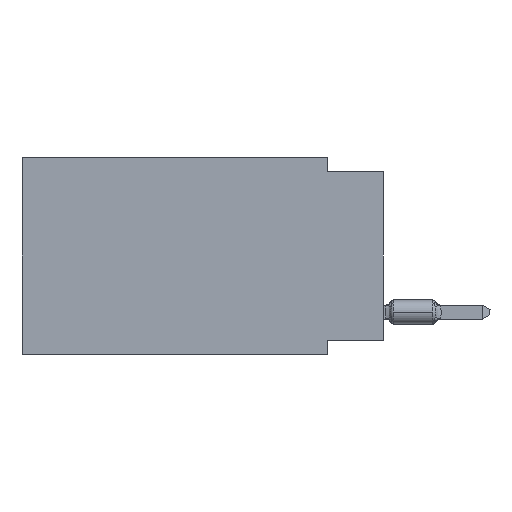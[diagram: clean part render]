
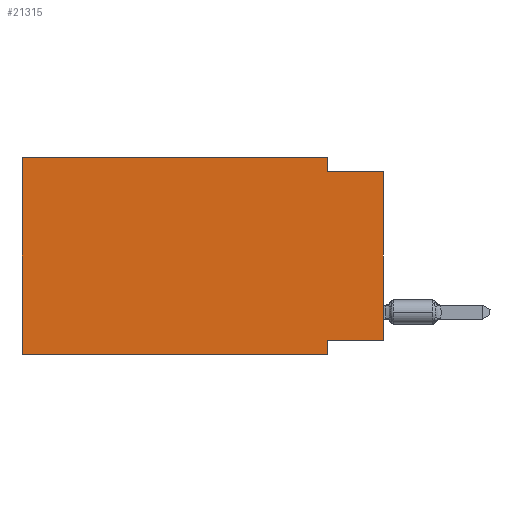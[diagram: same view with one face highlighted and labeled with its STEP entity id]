
A CAD part, left-side view. The second image highlights one B-rep face of the part: STEP entity #21315.
In plain terms, the highlighted planar face has unit normal (-1, 0, 0).
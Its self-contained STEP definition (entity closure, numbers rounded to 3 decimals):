
#63 = LINE ( 'NONE', #19021, #19771 ) ;
#945 = EDGE_CURVE ( 'NONE', #14390, #11680, #5071, .T. ) ;
#1278 = CARTESIAN_POINT ( 'NONE',  ( 0., 2.54, 0. ) ) ;
#1312 = LINE ( 'NONE', #8321, #14700 ) ;
#1321 = VECTOR ( 'NONE', #10752, 1000. ) ;
#1586 = CARTESIAN_POINT ( 'NONE',  ( 0., 0., -8.255 ) ) ;
#1684 = EDGE_CURVE ( 'NONE', #5217, #11494, #1312, .T. ) ;
#1720 = LINE ( 'NONE', #9074, #8133 ) ;
#1744 = DIRECTION ( 'NONE',  ( 0., -1., 0. ) ) ;
#2121 = VERTEX_POINT ( 'NONE', #20463 ) ;
#2567 = CARTESIAN_POINT ( 'NONE',  ( 0., 2.54, -8.89 ) ) ;
#4144 = CARTESIAN_POINT ( 'NONE',  ( 0., 16.383, 0. ) ) ;
#4177 = LINE ( 'NONE', #11512, #22068 ) ;
#4469 = PLANE ( 'NONE',  #6985 ) ;
#4640 = EDGE_CURVE ( 'NONE', #11680, #2121, #7028, .T. ) ;
#4866 = ORIENTED_EDGE ( 'NONE', *, *, #945, .F. ) ;
#5071 = LINE ( 'NONE', #1278, #19088 ) ;
#5217 = VERTEX_POINT ( 'NONE', #13508 ) ;
#6881 = DIRECTION ( 'NONE',  ( 0., -1., 0. ) ) ;
#6985 = AXIS2_PLACEMENT_3D ( 'NONE', #19994, #21599, #14577 ) ;
#7003 = LINE ( 'NONE', #8970, #14429 ) ;
#7018 = EDGE_CURVE ( 'NONE', #5217, #18439, #14177, .T. ) ;
#7028 = LINE ( 'NONE', #10482, #18991 ) ;
#7826 = VERTEX_POINT ( 'NONE', #1586 ) ;
#8072 = EDGE_LOOP ( 'NONE', ( #11065, #15018, #4866, #20286, #22439, #21670, #13181, #9648 ) ) ;
#8133 = VECTOR ( 'NONE', #6881, 1000. ) ;
#8321 = CARTESIAN_POINT ( 'NONE',  ( 0., 16.383, -8.89 ) ) ;
#8581 = DIRECTION ( 'NONE',  ( 0., 1., 0. ) ) ;
#8970 = CARTESIAN_POINT ( 'NONE',  ( 0., 2.54, -8.89 ) ) ;
#9074 = CARTESIAN_POINT ( 'NONE',  ( 0., 16.383, 0. ) ) ;
#9316 = FACE_OUTER_BOUND ( 'NONE', #8072, .T. ) ;
#9648 = ORIENTED_EDGE ( 'NONE', *, *, #9700, .F. ) ;
#9700 = EDGE_CURVE ( 'NONE', #7826, #15382, #63, .T. ) ;
#10275 = DIRECTION ( 'NONE',  ( 0., -1., 0. ) ) ;
#10283 = CARTESIAN_POINT ( 'NONE',  ( 0., 2.54, 0. ) ) ;
#10482 = CARTESIAN_POINT ( 'NONE',  ( 0., 0., -0.635 ) ) ;
#10752 = DIRECTION ( 'NONE',  ( 0., 0., 1. ) ) ;
#11065 = ORIENTED_EDGE ( 'NONE', *, *, #22175, .T. ) ;
#11494 = VERTEX_POINT ( 'NONE', #2567 ) ;
#11512 = CARTESIAN_POINT ( 'NONE',  ( 0., 0., 0. ) ) ;
#11680 = VERTEX_POINT ( 'NONE', #22098 ) ;
#12067 = DIRECTION ( 'NONE',  ( 0., 0., -1. ) ) ;
#13181 = ORIENTED_EDGE ( 'NONE', *, *, #15806, .F. ) ;
#13508 = CARTESIAN_POINT ( 'NONE',  ( 0., 16.383, -8.89 ) ) ;
#13555 = EDGE_CURVE ( 'NONE', #18439, #14390, #1720, .T. ) ;
#14177 = LINE ( 'NONE', #17755, #1321 ) ;
#14390 = VERTEX_POINT ( 'NONE', #10283 ) ;
#14429 = VECTOR ( 'NONE', #21027, 1000. ) ;
#14577 = DIRECTION ( 'NONE',  ( 0., 0., -1. ) ) ;
#14700 = VECTOR ( 'NONE', #10275, 1000. ) ;
#15018 = ORIENTED_EDGE ( 'NONE', *, *, #4640, .F. ) ;
#15382 = VERTEX_POINT ( 'NONE', #21794 ) ;
#15806 = EDGE_CURVE ( 'NONE', #15382, #11494, #7003, .T. ) ;
#17755 = CARTESIAN_POINT ( 'NONE',  ( 0., 16.383, 0. ) ) ;
#18439 = VERTEX_POINT ( 'NONE', #4144 ) ;
#18991 = VECTOR ( 'NONE', #1744, 1000. ) ;
#19021 = CARTESIAN_POINT ( 'NONE',  ( 0., 0., -8.255 ) ) ;
#19088 = VECTOR ( 'NONE', #12067, 1000. ) ;
#19771 = VECTOR ( 'NONE', #8581, 1000. ) ;
#19994 = CARTESIAN_POINT ( 'NONE',  ( 0., 16.383, 0. ) ) ;
#20286 = ORIENTED_EDGE ( 'NONE', *, *, #13555, .F. ) ;
#20463 = CARTESIAN_POINT ( 'NONE',  ( 0., 0., -0.635 ) ) ;
#21027 = DIRECTION ( 'NONE',  ( 0., 0., -1. ) ) ;
#21315 = ADVANCED_FACE ( 'NONE', ( #9316 ), #4469, .F. ) ;
#21599 = DIRECTION ( 'NONE',  ( 1., 0., 0. ) ) ;
#21670 = ORIENTED_EDGE ( 'NONE', *, *, #1684, .T. ) ;
#21794 = CARTESIAN_POINT ( 'NONE',  ( 0., 2.54, -8.255 ) ) ;
#22068 = VECTOR ( 'NONE', #22081, 1000. ) ;
#22081 = DIRECTION ( 'NONE',  ( 0., 0., 1. ) ) ;
#22098 = CARTESIAN_POINT ( 'NONE',  ( 0., 2.54, -0.635 ) ) ;
#22175 = EDGE_CURVE ( 'NONE', #7826, #2121, #4177, .T. ) ;
#22439 = ORIENTED_EDGE ( 'NONE', *, *, #7018, .F. ) ;
